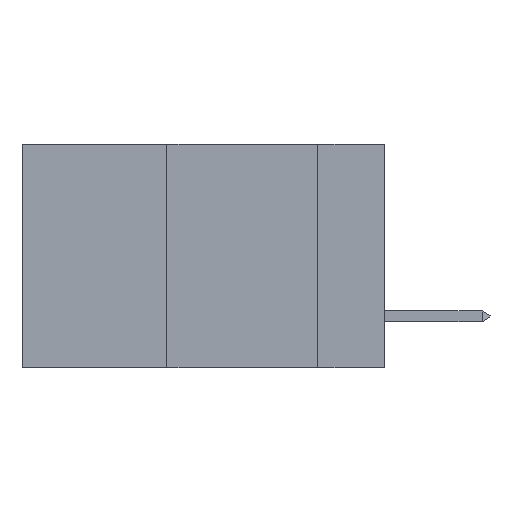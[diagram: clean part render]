
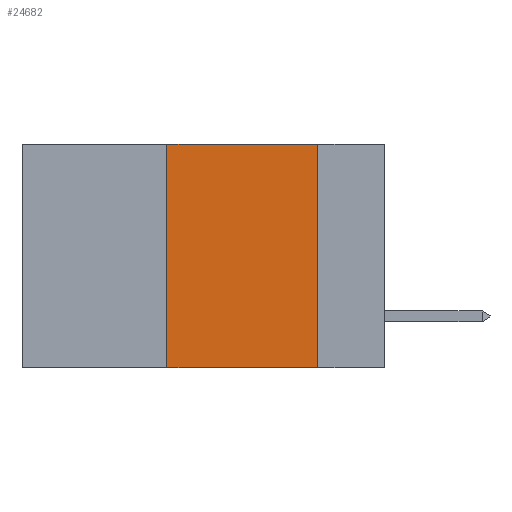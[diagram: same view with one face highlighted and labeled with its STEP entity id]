
A CAD part, left-side view. The second image highlights one B-rep face of the part: STEP entity #24682.
In plain terms, the highlighted planar face has unit normal (-1, 0, 0).
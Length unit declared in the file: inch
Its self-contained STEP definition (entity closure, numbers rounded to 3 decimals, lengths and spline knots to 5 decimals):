
#1415 = CARTESIAN_POINT ( 'NONE',  ( 0., 0.6, -0.37 ) ) ;
#2796 = VERTEX_POINT ( 'NONE', #7034 ) ;
#3077 = VECTOR ( 'NONE', #35472, 39.37008 ) ;
#3408 = ORIENTED_EDGE ( 'NONE', *, *, #9692, .F. ) ;
#5016 = EDGE_LOOP ( 'NONE', ( #27108, #6116, #3408, #20669 ) ) ;
#5198 = PLANE ( 'NONE',  #30658 ) ;
#6116 = ORIENTED_EDGE ( 'NONE', *, *, #37444, .F. ) ;
#6536 = VERTEX_POINT ( 'NONE', #38332 ) ;
#6905 = VECTOR ( 'NONE', #31248, 39.37008 ) ;
#7034 = CARTESIAN_POINT ( 'NONE',  ( 0., 0.11, -0.37 ) ) ;
#7461 = EDGE_CURVE ( 'NONE', #16680, #2796, #26879, .T. ) ;
#8822 = CARTESIAN_POINT ( 'NONE',  ( 0., 0.36, 0. ) ) ;
#9692 = EDGE_CURVE ( 'NONE', #16680, #21111, #30844, .T. ) ;
#10927 = VECTOR ( 'NONE', #22180, 39.37008 ) ;
#15455 = CARTESIAN_POINT ( 'NONE',  ( 0., 0.36, 0. ) ) ;
#16680 = VERTEX_POINT ( 'NONE', #36900 ) ;
#17450 = CARTESIAN_POINT ( 'NONE',  ( 0., 0.6, 0. ) ) ;
#17656 = DIRECTION ( 'NONE',  ( 1., 0., 0. ) ) ;
#19287 = DIRECTION ( 'NONE',  ( 0., 0., -1. ) ) ;
#20669 = ORIENTED_EDGE ( 'NONE', *, *, #7461, .T. ) ;
#21111 = VERTEX_POINT ( 'NONE', #15455 ) ;
#22180 = DIRECTION ( 'NONE',  ( 0., -1., 0. ) ) ;
#24682 = ADVANCED_FACE ( 'NONE', ( #38834 ), #5198, .F. ) ;
#26228 = VECTOR ( 'NONE', #19287, 39.37008 ) ;
#26879 = LINE ( 'NONE', #1415, #3077 ) ;
#27108 = ORIENTED_EDGE ( 'NONE', *, *, #28101, .F. ) ;
#28101 = EDGE_CURVE ( 'NONE', #6536, #2796, #34981, .T. ) ;
#29889 = DIRECTION ( 'NONE',  ( 0., 0., -1. ) ) ;
#30658 = AXIS2_PLACEMENT_3D ( 'NONE', #17450, #17656, #29889 ) ;
#30844 = LINE ( 'NONE', #8822, #6905 ) ;
#31248 = DIRECTION ( 'NONE',  ( 0., 0., 1. ) ) ;
#31526 = CARTESIAN_POINT ( 'NONE',  ( 0., 0.11, 0. ) ) ;
#34981 = LINE ( 'NONE', #31526, #26228 ) ;
#35472 = DIRECTION ( 'NONE',  ( 0., -1., 0. ) ) ;
#36900 = CARTESIAN_POINT ( 'NONE',  ( 0., 0.36, -0.37 ) ) ;
#37048 = CARTESIAN_POINT ( 'NONE',  ( 0., 0.6, 0. ) ) ;
#37444 = EDGE_CURVE ( 'NONE', #21111, #6536, #37855, .T. ) ;
#37855 = LINE ( 'NONE', #37048, #10927 ) ;
#38332 = CARTESIAN_POINT ( 'NONE',  ( 0., 0.11, 0. ) ) ;
#38834 = FACE_OUTER_BOUND ( 'NONE', #5016, .T. ) ;
